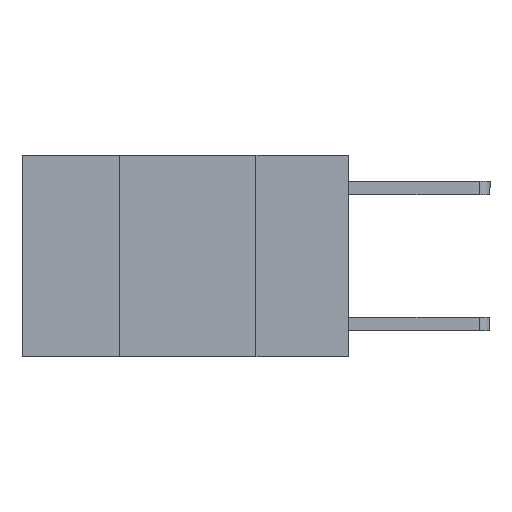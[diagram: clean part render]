
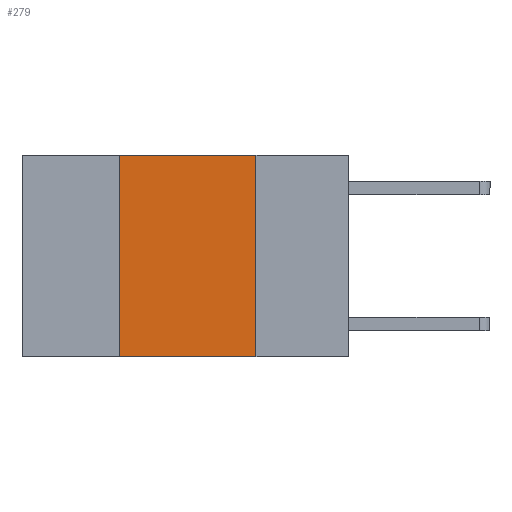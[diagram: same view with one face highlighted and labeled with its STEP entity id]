
A CAD part, left-side view. The second image highlights one B-rep face of the part: STEP entity #279.
In plain terms, the highlighted planar face has unit normal (-1, 0, 0).
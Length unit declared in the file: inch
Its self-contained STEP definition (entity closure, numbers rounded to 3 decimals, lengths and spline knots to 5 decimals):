
#218 = AXIS2_PLACEMENT_3D ( 'NONE', #1818, #5311, #8644 ) ;
#279 = ADVANCED_FACE ( 'NONE', ( #5870 ), #9142, .F. ) ;
#420 = CARTESIAN_POINT ( 'NONE',  ( 0., 0.42, 0. ) ) ;
#456 = CARTESIAN_POINT ( 'NONE',  ( 0., 0.42, -0.37 ) ) ;
#893 = EDGE_CURVE ( 'NONE', #9837, #8055, #6591, .T. ) ;
#1038 = VECTOR ( 'NONE', #8107, 39.37008 ) ;
#1448 = ORIENTED_EDGE ( 'NONE', *, *, #9061, .F. ) ;
#1818 = CARTESIAN_POINT ( 'NONE',  ( 0., 0.6, 0. ) ) ;
#1874 = CARTESIAN_POINT ( 'NONE',  ( 0., 0.17, 0. ) ) ;
#2768 = VECTOR ( 'NONE', #9699, 39.37008 ) ;
#3167 = CARTESIAN_POINT ( 'NONE',  ( 0., 0.6, -0.37 ) ) ;
#3241 = ORIENTED_EDGE ( 'NONE', *, *, #893, .T. ) ;
#3288 = CARTESIAN_POINT ( 'NONE',  ( 0., 0.6, 0. ) ) ;
#3351 = VECTOR ( 'NONE', #5097, 39.37008 ) ;
#3672 = LINE ( 'NONE', #1874, #3351 ) ;
#3752 = EDGE_LOOP ( 'NONE', ( #4035, #7301, #1448, #3241 ) ) ;
#3843 = EDGE_CURVE ( 'NONE', #7658, #9881, #6607, .T. ) ;
#3868 = LINE ( 'NONE', #8743, #1038 ) ;
#4035 = ORIENTED_EDGE ( 'NONE', *, *, #5427, .F. ) ;
#5009 = VECTOR ( 'NONE', #8369, 39.37008 ) ;
#5097 = DIRECTION ( 'NONE',  ( 0., 0., -1. ) ) ;
#5311 = DIRECTION ( 'NONE',  ( 1., 0., 0. ) ) ;
#5334 = CARTESIAN_POINT ( 'NONE',  ( 0., 0.17, 0. ) ) ;
#5427 = EDGE_CURVE ( 'NONE', #9881, #8055, #3672, .T. ) ;
#5870 = FACE_OUTER_BOUND ( 'NONE', #3752, .T. ) ;
#6478 = CARTESIAN_POINT ( 'NONE',  ( 0., 0.17, -0.37 ) ) ;
#6591 = LINE ( 'NONE', #3167, #2768 ) ;
#6607 = LINE ( 'NONE', #3288, #5009 ) ;
#7301 = ORIENTED_EDGE ( 'NONE', *, *, #3843, .F. ) ;
#7658 = VERTEX_POINT ( 'NONE', #420 ) ;
#8055 = VERTEX_POINT ( 'NONE', #6478 ) ;
#8107 = DIRECTION ( 'NONE',  ( 0., 0., 1. ) ) ;
#8369 = DIRECTION ( 'NONE',  ( 0., -1., 0. ) ) ;
#8644 = DIRECTION ( 'NONE',  ( 0., 0., -1. ) ) ;
#8743 = CARTESIAN_POINT ( 'NONE',  ( 0., 0.42, 0. ) ) ;
#9061 = EDGE_CURVE ( 'NONE', #9837, #7658, #3868, .T. ) ;
#9142 = PLANE ( 'NONE',  #218 ) ;
#9699 = DIRECTION ( 'NONE',  ( 0., -1., 0. ) ) ;
#9837 = VERTEX_POINT ( 'NONE', #456 ) ;
#9881 = VERTEX_POINT ( 'NONE', #5334 ) ;
